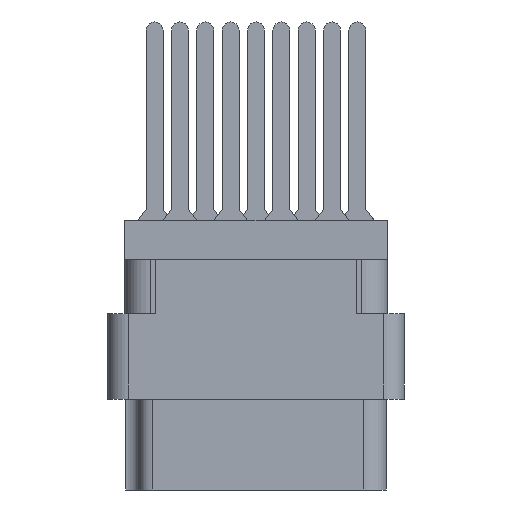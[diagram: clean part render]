
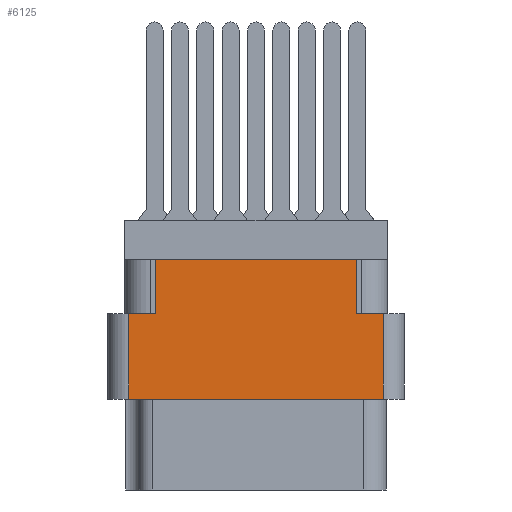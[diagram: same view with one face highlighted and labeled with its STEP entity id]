
A CAD part, left-side view. The second image highlights one B-rep face of the part: STEP entity #6125.
In plain terms, the highlighted planar face has unit normal (-1, 0, 0).
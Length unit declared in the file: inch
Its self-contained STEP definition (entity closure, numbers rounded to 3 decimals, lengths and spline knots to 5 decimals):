
#541 = EDGE_LOOP ( 'NONE', ( #21528, #13469, #14364, #5664, #22952, #32518, #33843, #6310 ) ) ;
#574 = EDGE_CURVE ( 'NONE', #9292, #29172, #9072, .T. ) ;
#2893 = CARTESIAN_POINT ( 'NONE',  ( -1., 0.376, -0.798 ) ) ;
#3219 = CARTESIAN_POINT ( 'NONE',  ( -1., 0.296, -0.277 ) ) ;
#3410 = LINE ( 'NONE', #25784, #34360 ) ;
#3467 = VERTEX_POINT ( 'NONE', #29793 ) ;
#4145 = DIRECTION ( 'NONE',  ( 0., 1., 0. ) ) ;
#5664 = ORIENTED_EDGE ( 'NONE', *, *, #25056, .T. ) ;
#6034 = EDGE_CURVE ( 'NONE', #23464, #9292, #3410, .T. ) ;
#6125 = ADVANCED_FACE ( 'NONE', ( #24532 ), #22594, .T. ) ;
#6291 = LINE ( 'NONE', #24264, #28315 ) ;
#6310 = ORIENTED_EDGE ( 'NONE', *, *, #6034, .F. ) ;
#6347 = CARTESIAN_POINT ( 'NONE',  ( -1., 0.376, -0.277 ) ) ;
#7011 = VECTOR ( 'NONE', #23545, 39.37008 ) ;
#7198 = EDGE_CURVE ( 'NONE', #23033, #26417, #38469, .T. ) ;
#8078 = DIRECTION ( 'NONE',  ( 0., -1., 0. ) ) ;
#8282 = EDGE_CURVE ( 'NONE', #3467, #27974, #19693, .T. ) ;
#9072 = LINE ( 'NONE', #26233, #26413 ) ;
#9292 = VERTEX_POINT ( 'NONE', #18387 ) ;
#11274 = DIRECTION ( 'NONE',  ( 0., -1., 0. ) ) ;
#11712 = CARTESIAN_POINT ( 'NONE',  ( -1., -0.376, -0.277 ) ) ;
#12432 = EDGE_CURVE ( 'NONE', #31960, #26417, #32611, .T. ) ;
#13403 = EDGE_CURVE ( 'NONE', #3467, #29172, #6291, .T. ) ;
#13469 = ORIENTED_EDGE ( 'NONE', *, *, #12432, .T. ) ;
#13812 = CARTESIAN_POINT ( 'NONE',  ( -1., -0.296, -0.117 ) ) ;
#13846 = DIRECTION ( 'NONE',  ( 0., 0., 1. ) ) ;
#14364 = ORIENTED_EDGE ( 'NONE', *, *, #7198, .F. ) ;
#14827 = DIRECTION ( 'NONE',  ( 0., 0., -1. ) ) ;
#15626 = LINE ( 'NONE', #23037, #18459 ) ;
#16960 = VECTOR ( 'NONE', #4145, 39.37008 ) ;
#18387 = CARTESIAN_POINT ( 'NONE',  ( -1., 0.296, -0.117 ) ) ;
#18459 = VECTOR ( 'NONE', #8078, 39.37008 ) ;
#19646 = DIRECTION ( 'NONE',  ( 0., 0., 1. ) ) ;
#19693 = LINE ( 'NONE', #20540, #7011 ) ;
#20540 = CARTESIAN_POINT ( 'NONE',  ( -1., 0., -0.277 ) ) ;
#21528 = ORIENTED_EDGE ( 'NONE', *, *, #31747, .F. ) ;
#21874 = CARTESIAN_POINT ( 'NONE',  ( -1., 0., -0.529 ) ) ;
#22354 = DIRECTION ( 'NONE',  ( 0., 0., 1. ) ) ;
#22594 = PLANE ( 'NONE',  #33362 ) ;
#22952 = ORIENTED_EDGE ( 'NONE', *, *, #8282, .F. ) ;
#23033 = VERTEX_POINT ( 'NONE', #30248 ) ;
#23037 = CARTESIAN_POINT ( 'NONE',  ( -1., 0., -0.277 ) ) ;
#23464 = VERTEX_POINT ( 'NONE', #3219 ) ;
#23545 = DIRECTION ( 'NONE',  ( 0., -1., 0. ) ) ;
#24264 = CARTESIAN_POINT ( 'NONE',  ( -1., -0.296, -0.277 ) ) ;
#24532 = FACE_OUTER_BOUND ( 'NONE', #541, .T. ) ;
#25056 = EDGE_CURVE ( 'NONE', #23033, #27974, #37285, .T. ) ;
#25784 = CARTESIAN_POINT ( 'NONE',  ( -1., 0.296, -0.277 ) ) ;
#26078 = VECTOR ( 'NONE', #19646, 39.37008 ) ;
#26233 = CARTESIAN_POINT ( 'NONE',  ( -1., 0.438, -0.117 ) ) ;
#26413 = VECTOR ( 'NONE', #11274, 39.37008 ) ;
#26417 = VERTEX_POINT ( 'NONE', #28349 ) ;
#27974 = VERTEX_POINT ( 'NONE', #11712 ) ;
#28315 = VECTOR ( 'NONE', #32608, 39.37008 ) ;
#28349 = CARTESIAN_POINT ( 'NONE',  ( -1., 0.376, -0.529 ) ) ;
#28866 = VECTOR ( 'NONE', #14827, 39.37008 ) ;
#29172 = VERTEX_POINT ( 'NONE', #13812 ) ;
#29793 = CARTESIAN_POINT ( 'NONE',  ( -1., -0.296, -0.277 ) ) ;
#30248 = CARTESIAN_POINT ( 'NONE',  ( -1., -0.376, -0.529 ) ) ;
#31348 = CARTESIAN_POINT ( 'NONE',  ( -1., -0.438, -0.798 ) ) ;
#31747 = EDGE_CURVE ( 'NONE', #31960, #23464, #15626, .T. ) ;
#31960 = VERTEX_POINT ( 'NONE', #6347 ) ;
#32518 = ORIENTED_EDGE ( 'NONE', *, *, #13403, .T. ) ;
#32608 = DIRECTION ( 'NONE',  ( 0., 0., 1. ) ) ;
#32611 = LINE ( 'NONE', #2893, #28866 ) ;
#33362 = AXIS2_PLACEMENT_3D ( 'NONE', #31348, #37610, #22354 ) ;
#33843 = ORIENTED_EDGE ( 'NONE', *, *, #574, .F. ) ;
#34360 = VECTOR ( 'NONE', #13846, 39.37008 ) ;
#37285 = LINE ( 'NONE', #37805, #26078 ) ;
#37610 = DIRECTION ( 'NONE',  ( -1., 0., 0. ) ) ;
#37805 = CARTESIAN_POINT ( 'NONE',  ( -1., -0.376, -0.798 ) ) ;
#38469 = LINE ( 'NONE', #21874, #16960 ) ;
